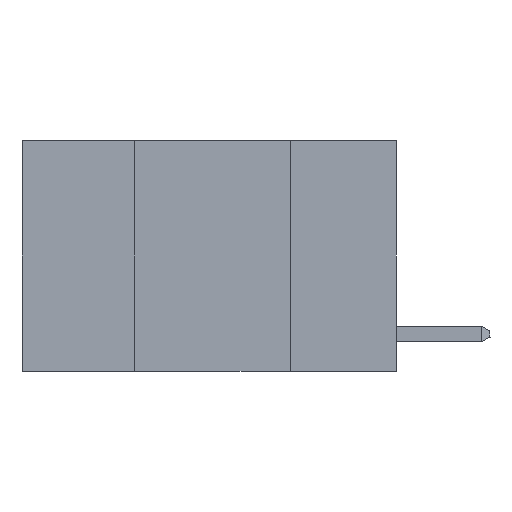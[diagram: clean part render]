
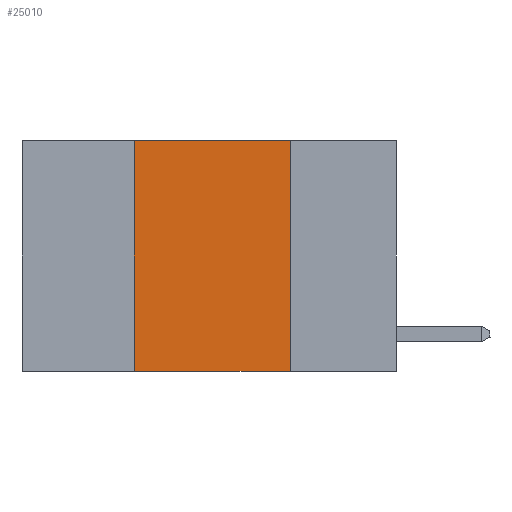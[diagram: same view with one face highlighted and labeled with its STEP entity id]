
A CAD part, left-side view. The second image highlights one B-rep face of the part: STEP entity #25010.
In plain terms, the highlighted planar face has unit normal (-1, 0, 0).
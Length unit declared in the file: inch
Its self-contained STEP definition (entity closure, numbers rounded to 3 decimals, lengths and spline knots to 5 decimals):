
#327 = ORIENTED_EDGE ( 'NONE', *, *, #13969, .F. ) ;
#1478 = AXIS2_PLACEMENT_3D ( 'NONE', #23447, #5337, #19514 ) ;
#1667 = VECTOR ( 'NONE', #4873, 39.37008 ) ;
#3554 = VERTEX_POINT ( 'NONE', #15145 ) ;
#3683 = ORIENTED_EDGE ( 'NONE', *, *, #22330, .F. ) ;
#3692 = VERTEX_POINT ( 'NONE', #19587 ) ;
#3939 = VECTOR ( 'NONE', #6051, 39.37008 ) ;
#4873 = DIRECTION ( 'NONE',  ( 0., 0., -1. ) ) ;
#5337 = DIRECTION ( 'NONE',  ( 1., 0., 0. ) ) ;
#6051 = DIRECTION ( 'NONE',  ( 0., -1., 0. ) ) ;
#7301 = EDGE_LOOP ( 'NONE', ( #8751, #3683, #327, #25319 ) ) ;
#7505 = FACE_OUTER_BOUND ( 'NONE', #7301, .T. ) ;
#7592 = VECTOR ( 'NONE', #22976, 39.37008 ) ;
#8146 = CARTESIAN_POINT ( 'NONE',  ( 0., 0.17, 0. ) ) ;
#8751 = ORIENTED_EDGE ( 'NONE', *, *, #22639, .F. ) ;
#9561 = VERTEX_POINT ( 'NONE', #24839 ) ;
#9927 = EDGE_CURVE ( 'NONE', #3554, #9561, #11753, .T. ) ;
#11753 = LINE ( 'NONE', #25937, #22528 ) ;
#13860 = DIRECTION ( 'NONE',  ( 0., -1., 0. ) ) ;
#13969 = EDGE_CURVE ( 'NONE', #3554, #3692, #23691, .T. ) ;
#15145 = CARTESIAN_POINT ( 'NONE',  ( 0., 0.42, -0.37 ) ) ;
#17459 = PLANE ( 'NONE',  #1478 ) ;
#19054 = CARTESIAN_POINT ( 'NONE',  ( 0., 0.17, 0. ) ) ;
#19514 = DIRECTION ( 'NONE',  ( 0., 0., -1. ) ) ;
#19587 = CARTESIAN_POINT ( 'NONE',  ( 0., 0.42, 0. ) ) ;
#20129 = LINE ( 'NONE', #26141, #3939 ) ;
#20981 = CARTESIAN_POINT ( 'NONE',  ( 0., 0.42, 0. ) ) ;
#22330 = EDGE_CURVE ( 'NONE', #3692, #25867, #20129, .T. ) ;
#22528 = VECTOR ( 'NONE', #13860, 39.37008 ) ;
#22639 = EDGE_CURVE ( 'NONE', #25867, #9561, #23850, .T. ) ;
#22976 = DIRECTION ( 'NONE',  ( 0., 0., 1. ) ) ;
#23447 = CARTESIAN_POINT ( 'NONE',  ( 0., 0.6, 0. ) ) ;
#23691 = LINE ( 'NONE', #20981, #7592 ) ;
#23850 = LINE ( 'NONE', #19054, #1667 ) ;
#24839 = CARTESIAN_POINT ( 'NONE',  ( 0., 0.17, -0.37 ) ) ;
#25010 = ADVANCED_FACE ( 'NONE', ( #7505 ), #17459, .F. ) ;
#25319 = ORIENTED_EDGE ( 'NONE', *, *, #9927, .T. ) ;
#25867 = VERTEX_POINT ( 'NONE', #8146 ) ;
#25937 = CARTESIAN_POINT ( 'NONE',  ( 0., 0.6, -0.37 ) ) ;
#26141 = CARTESIAN_POINT ( 'NONE',  ( 0., 0.6, 0. ) ) ;
